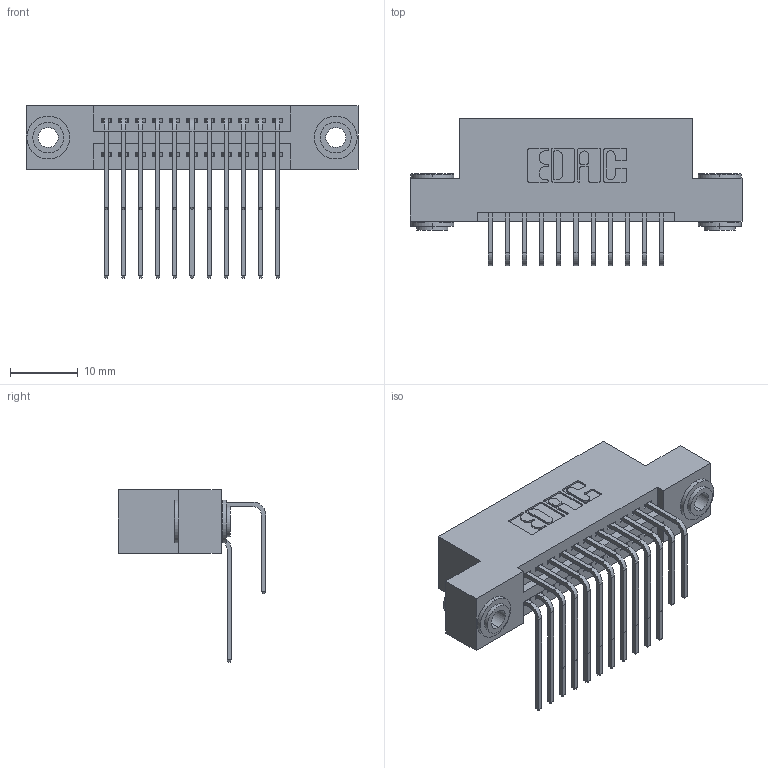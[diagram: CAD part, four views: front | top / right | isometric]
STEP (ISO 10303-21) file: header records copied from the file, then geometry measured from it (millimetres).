
FILE_DESCRIPTION (( 'STEP AP203' ), '1' );
FILE_NAME ('395-022-558-203.STEP', '2018-11-08T05:48:31', ( '' ), ( '' ), 'SwSTEP 2.0', 'SolidWorks 2016', '' );
FILE_SCHEMA (( 'CONFIG_CONTROL_DESIGN' ));
Length unit declared in the file: inch
Products named in the file (5): 345-292-001_558 559 Tail - 1; 345-292-001_558 Tail - 2; 395-022-558-203; 345 Part_Flush Mounting Lugs - 0.156 Dia-TH; 345-250-002_345-250-002-102
Assembly tree (25 placements, depth 2):
  395-022-558-203
    345 Part_Flush Mounting Lugs - 0.156 Dia-TH
    345-292-001_558 559 Tail - 1  x11
    345-292-001_558 Tail - 2  x11
    345-250-002_345-250-002-102  x2
Bounding box: 49.15 x 21.83 x 25.53 mm (x, y, z)
Volume: 4632.9 mm3; surface area: 7049.5 mm2
Topology: 25 solids, 25 shells, 1308 faces, 3827 edges, 2518 vertices
Faces by surface type: plane 860, cylinder 440, cone 8
Entity records: 15106 total; most frequent: CARTESIAN_POINT 2582, ORIENTED_EDGE 2458, DIRECTION 2319, EDGE_CURVE 1229, VECTOR 989, LINE 989, VERTEX_POINT 814, AXIS2_PLACEMENT_3D 665
